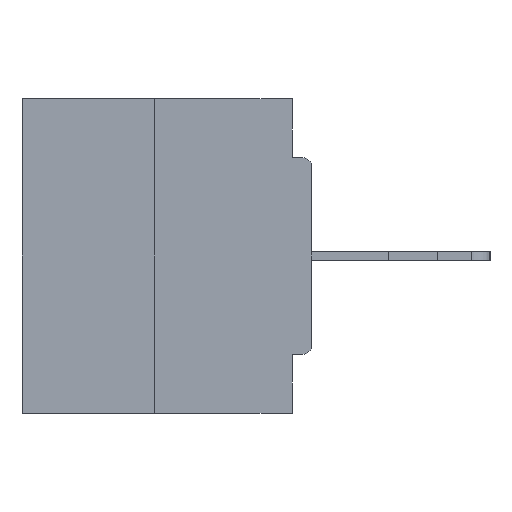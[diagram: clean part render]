
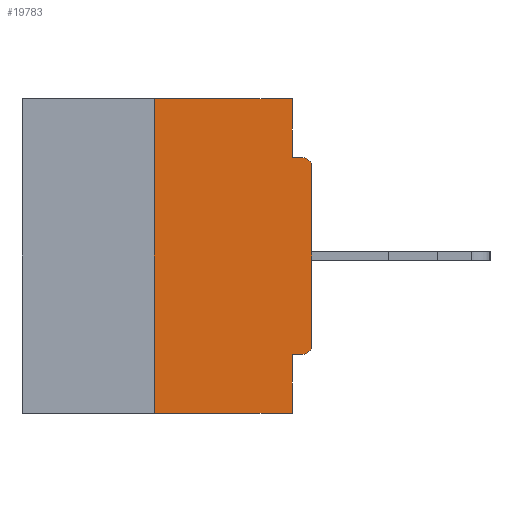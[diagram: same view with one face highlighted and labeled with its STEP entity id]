
A CAD part, left-side view. The second image highlights one B-rep face of the part: STEP entity #19783.
In plain terms, the highlighted planar face has unit normal (-1, 0, 0).
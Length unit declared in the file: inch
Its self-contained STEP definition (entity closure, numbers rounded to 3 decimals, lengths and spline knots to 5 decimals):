
#19 = LINE ( 'NONE', #12636, #15572 ) ;
#94 = DIRECTION ( 'NONE',  ( 0., 1., 0. ) ) ;
#477 = CARTESIAN_POINT ( 'NONE',  ( 0., 0.46, 0. ) ) ;
#1134 = FACE_OUTER_BOUND ( 'NONE', #33168, .T. ) ;
#1468 = VERTEX_POINT ( 'NONE', #1954 ) ;
#1513 = VERTEX_POINT ( 'NONE', #22059 ) ;
#1675 = DIRECTION ( 'NONE',  ( 0., 0., 1. ) ) ;
#1954 = CARTESIAN_POINT ( 'NONE',  ( 0., 0.25, 0. ) ) ;
#2068 = CARTESIAN_POINT ( 'NONE',  ( 0., 0.031, 0. ) ) ;
#2128 = CIRCLE ( 'NONE', #27155, 0.015 ) ;
#2538 = EDGE_CURVE ( 'NONE', #4238, #4649, #28333, .T. ) ;
#3626 = DIRECTION ( 'NONE',  ( 0., 0., -1. ) ) ;
#4238 = VERTEX_POINT ( 'NONE', #18876 ) ;
#4649 = VERTEX_POINT ( 'NONE', #35094 ) ;
#5018 = EDGE_CURVE ( 'NONE', #4238, #7866, #36940, .T. ) ;
#5221 = ORIENTED_EDGE ( 'NONE', *, *, #25054, .F. ) ;
#6679 = ORIENTED_EDGE ( 'NONE', *, *, #30706, .T. ) ;
#7409 = LINE ( 'NONE', #11899, #22549 ) ;
#7475 = LINE ( 'NONE', #16267, #12824 ) ;
#7866 = VERTEX_POINT ( 'NONE', #28940 ) ;
#7933 = DIRECTION ( 'NONE',  ( 0., -1., 0. ) ) ;
#8149 = ORIENTED_EDGE ( 'NONE', *, *, #36440, .F. ) ;
#8241 = EDGE_CURVE ( 'NONE', #19601, #32434, #2128, .T. ) ;
#8372 = EDGE_CURVE ( 'NONE', #4649, #13727, #7475, .T. ) ;
#8720 = LINE ( 'NONE', #31631, #23762 ) ;
#8982 = CARTESIAN_POINT ( 'NONE',  ( 0., 0., -0.1085 ) ) ;
#10788 = LINE ( 'NONE', #20001, #25752 ) ;
#11597 = ORIENTED_EDGE ( 'NONE', *, *, #29905, .F. ) ;
#11899 = CARTESIAN_POINT ( 'NONE',  ( 0., 0.031, 0. ) ) ;
#12063 = ORIENTED_EDGE ( 'NONE', *, *, #5018, .T. ) ;
#12636 = CARTESIAN_POINT ( 'NONE',  ( 0., 0., 0. ) ) ;
#12815 = DIRECTION ( 'NONE',  ( -1., 0., 0. ) ) ;
#12824 = VECTOR ( 'NONE', #34275, 39.37008 ) ;
#13727 = VERTEX_POINT ( 'NONE', #20895 ) ;
#15321 = CARTESIAN_POINT ( 'NONE',  ( 0., 0., -0.4065 ) ) ;
#15572 = VECTOR ( 'NONE', #15688, 39.37008 ) ;
#15688 = DIRECTION ( 'NONE',  ( 0., 0., 1. ) ) ;
#16182 = LINE ( 'NONE', #32109, #23110 ) ;
#16267 = CARTESIAN_POINT ( 'NONE',  ( 0., 0.031, -0.5 ) ) ;
#17237 = ORIENTED_EDGE ( 'NONE', *, *, #22678, .T. ) ;
#18876 = CARTESIAN_POINT ( 'NONE',  ( 0., 0.015, -0.4065 ) ) ;
#19545 = VERTEX_POINT ( 'NONE', #23697 ) ;
#19601 = VERTEX_POINT ( 'NONE', #8982 ) ;
#19783 = ADVANCED_FACE ( 'NONE', ( #1134 ), #36839, .F. ) ;
#20001 = CARTESIAN_POINT ( 'NONE',  ( 0., 0.46, 0. ) ) ;
#20895 = CARTESIAN_POINT ( 'NONE',  ( 0., 0.031, -0.5 ) ) ;
#21323 = LINE ( 'NONE', #33108, #28349 ) ;
#21860 = DIRECTION ( 'NONE',  ( 1., 0., 0. ) ) ;
#22059 = CARTESIAN_POINT ( 'NONE',  ( 0., 0.25, -0.5 ) ) ;
#22549 = VECTOR ( 'NONE', #32857, 39.37008 ) ;
#22678 = EDGE_CURVE ( 'NONE', #1513, #13727, #21323, .T. ) ;
#23048 = DIRECTION ( 'NONE',  ( 0., 0., -1. ) ) ;
#23083 = DIRECTION ( 'NONE',  ( -1., 0., 0. ) ) ;
#23110 = VECTOR ( 'NONE', #1675, 39.37008 ) ;
#23171 = CARTESIAN_POINT ( 'NONE',  ( 0., 0.015, -0.3915 ) ) ;
#23697 = CARTESIAN_POINT ( 'NONE',  ( 0., 0.031, -0.0935 ) ) ;
#23762 = VECTOR ( 'NONE', #34607, 39.37008 ) ;
#24130 = DIRECTION ( 'NONE',  ( 0., -1., 0. ) ) ;
#25054 = EDGE_CURVE ( 'NONE', #1468, #38600, #10788, .T. ) ;
#25294 = AXIS2_PLACEMENT_3D ( 'NONE', #23171, #23083, #23048 ) ;
#25752 = VECTOR ( 'NONE', #7933, 39.37008 ) ;
#26433 = VECTOR ( 'NONE', #94, 39.37008 ) ;
#27155 = AXIS2_PLACEMENT_3D ( 'NONE', #30771, #12815, #33754 ) ;
#28333 = LINE ( 'NONE', #15321, #26433 ) ;
#28349 = VECTOR ( 'NONE', #24130, 39.37008 ) ;
#28940 = CARTESIAN_POINT ( 'NONE',  ( 0., 0., -0.3915 ) ) ;
#29905 = EDGE_CURVE ( 'NONE', #38600, #19545, #7409, .T. ) ;
#30057 = CARTESIAN_POINT ( 'NONE',  ( 0., 0.015, -0.0935 ) ) ;
#30509 = AXIS2_PLACEMENT_3D ( 'NONE', #477, #21860, #3626 ) ;
#30706 = EDGE_CURVE ( 'NONE', #7866, #19601, #19, .T. ) ;
#30771 = CARTESIAN_POINT ( 'NONE',  ( 0., 0.015, -0.1085 ) ) ;
#30822 = ORIENTED_EDGE ( 'NONE', *, *, #8241, .T. ) ;
#31631 = CARTESIAN_POINT ( 'NONE',  ( 0., 0., -0.0935 ) ) ;
#31774 = ORIENTED_EDGE ( 'NONE', *, *, #34543, .F. ) ;
#32109 = CARTESIAN_POINT ( 'NONE',  ( 0., 0.25, 0. ) ) ;
#32434 = VERTEX_POINT ( 'NONE', #30057 ) ;
#32857 = DIRECTION ( 'NONE',  ( 0., 0., -1. ) ) ;
#33108 = CARTESIAN_POINT ( 'NONE',  ( 0., 0.46, -0.5 ) ) ;
#33131 = ORIENTED_EDGE ( 'NONE', *, *, #8372, .F. ) ;
#33168 = EDGE_LOOP ( 'NONE', ( #5221, #8149, #17237, #33131, #35012, #12063, #6679, #30822, #31774, #11597 ) ) ;
#33754 = DIRECTION ( 'NONE',  ( 0., 0., -1. ) ) ;
#34275 = DIRECTION ( 'NONE',  ( 0., 0., -1. ) ) ;
#34543 = EDGE_CURVE ( 'NONE', #19545, #32434, #8720, .T. ) ;
#34607 = DIRECTION ( 'NONE',  ( 0., -1., 0. ) ) ;
#35012 = ORIENTED_EDGE ( 'NONE', *, *, #2538, .F. ) ;
#35094 = CARTESIAN_POINT ( 'NONE',  ( 0., 0.031, -0.4065 ) ) ;
#36440 = EDGE_CURVE ( 'NONE', #1513, #1468, #16182, .T. ) ;
#36839 = PLANE ( 'NONE',  #30509 ) ;
#36940 = CIRCLE ( 'NONE', #25294, 0.015 ) ;
#38600 = VERTEX_POINT ( 'NONE', #2068 ) ;
